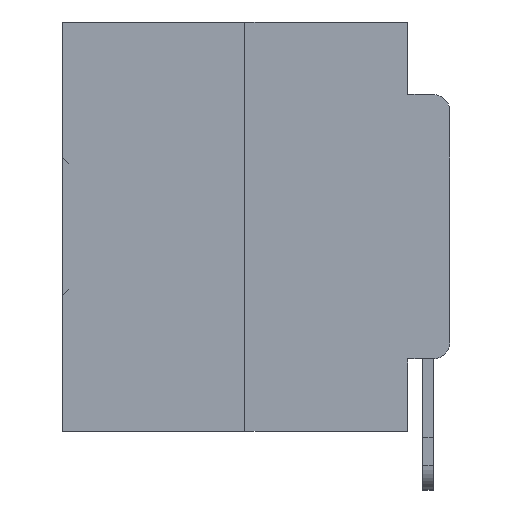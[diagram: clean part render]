
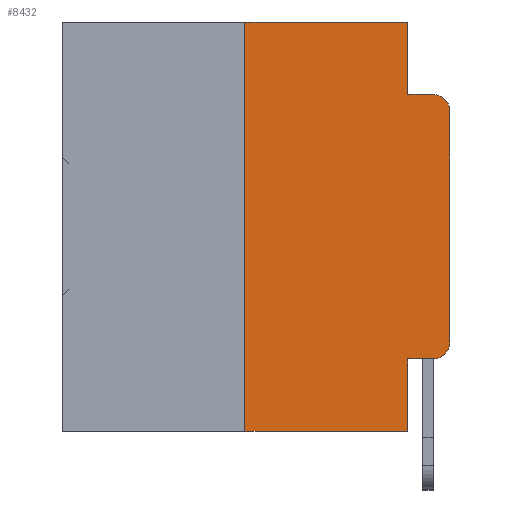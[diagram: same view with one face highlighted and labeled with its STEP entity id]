
A CAD part, left-side view. The second image highlights one B-rep face of the part: STEP entity #8432.
In plain terms, the highlighted planar face has unit normal (-1, 0, 0).
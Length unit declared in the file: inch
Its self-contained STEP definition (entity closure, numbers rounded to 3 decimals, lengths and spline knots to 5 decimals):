
#310 = CARTESIAN_POINT ( 'NONE',  ( 0., 0.473, 0. ) ) ;
#440 = DIRECTION ( 'NONE',  ( 0., 0., -1. ) ) ;
#893 = CARTESIAN_POINT ( 'NONE',  ( 0., 0., 0. ) ) ;
#908 = VERTEX_POINT ( 'NONE', #3097 ) ;
#1462 = CARTESIAN_POINT ( 'NONE',  ( 0., 0.02, -0.1085 ) ) ;
#2169 = ORIENTED_EDGE ( 'NONE', *, *, #18929, .F. ) ;
#3097 = CARTESIAN_POINT ( 'NONE',  ( 0., 0., -0.3915 ) ) ;
#3182 = DIRECTION ( 'NONE',  ( 1., 0., 0. ) ) ;
#3212 = DIRECTION ( 'NONE',  ( 0., -1., 0. ) ) ;
#3274 = ORIENTED_EDGE ( 'NONE', *, *, #28466, .T. ) ;
#3740 = DIRECTION ( 'NONE',  ( 0., 0., 1. ) ) ;
#4311 = DIRECTION ( 'NONE',  ( 0., 0., -1. ) ) ;
#4549 = CARTESIAN_POINT ( 'NONE',  ( 0., 0.051, 0. ) ) ;
#4976 = ORIENTED_EDGE ( 'NONE', *, *, #17083, .F. ) ;
#5153 = VERTEX_POINT ( 'NONE', #35256 ) ;
#5606 = DIRECTION ( 'NONE',  ( 0., -1., 0. ) ) ;
#5955 = CARTESIAN_POINT ( 'NONE',  ( 0., 0.25, 0. ) ) ;
#6010 = LINE ( 'NONE', #14475, #27039 ) ;
#7073 = CARTESIAN_POINT ( 'NONE',  ( 0., 0.051, -0.0885 ) ) ;
#7370 = DIRECTION ( 'NONE',  ( -1., 0., 0. ) ) ;
#7690 = ORIENTED_EDGE ( 'NONE', *, *, #12234, .F. ) ;
#8172 = VERTEX_POINT ( 'NONE', #31947 ) ;
#8432 = ADVANCED_FACE ( 'NONE', ( #31484 ), #33073, .F. ) ;
#9915 = DIRECTION ( 'NONE',  ( 0., -1., 0. ) ) ;
#10198 = ORIENTED_EDGE ( 'NONE', *, *, #22091, .T. ) ;
#10309 = EDGE_CURVE ( 'NONE', #22016, #10993, #26444, .T. ) ;
#10993 = VERTEX_POINT ( 'NONE', #33402 ) ;
#11069 = VECTOR ( 'NONE', #3212, 39.37008 ) ;
#11459 = DIRECTION ( 'NONE',  ( 0., 0., -1. ) ) ;
#11576 = DIRECTION ( 'NONE',  ( 0., 0., 1. ) ) ;
#11639 = ORIENTED_EDGE ( 'NONE', *, *, #15289, .T. ) ;
#12204 = ORIENTED_EDGE ( 'NONE', *, *, #10309, .T. ) ;
#12234 = EDGE_CURVE ( 'NONE', #34002, #23517, #28386, .T. ) ;
#12989 = CIRCLE ( 'NONE', #17070, 0.02 ) ;
#12990 = ORIENTED_EDGE ( 'NONE', *, *, #20644, .F. ) ;
#13266 = CARTESIAN_POINT ( 'NONE',  ( 0., 0.473, -0.5 ) ) ;
#13388 = CARTESIAN_POINT ( 'NONE',  ( 0., 0.051, -0.0885 ) ) ;
#13579 = VERTEX_POINT ( 'NONE', #4549 ) ;
#13599 = LINE ( 'NONE', #27549, #34909 ) ;
#14023 = VECTOR ( 'NONE', #9915, 39.37008 ) ;
#14372 = VECTOR ( 'NONE', #3740, 39.37008 ) ;
#14475 = CARTESIAN_POINT ( 'NONE',  ( 0., 0.051, 0. ) ) ;
#15289 = EDGE_CURVE ( 'NONE', #908, #8172, #28723, .T. ) ;
#16059 = DIRECTION ( 'NONE',  ( 0., -1., 0. ) ) ;
#16426 = EDGE_CURVE ( 'NONE', #13579, #34002, #6010, .T. ) ;
#17070 = AXIS2_PLACEMENT_3D ( 'NONE', #23861, #7370, #11459 ) ;
#17083 = EDGE_CURVE ( 'NONE', #22016, #24878, #22803, .T. ) ;
#17811 = EDGE_CURVE ( 'NONE', #8172, #23517, #33086, .T. ) ;
#18929 = EDGE_CURVE ( 'NONE', #23051, #5153, #27285, .T. ) ;
#19375 = AXIS2_PLACEMENT_3D ( 'NONE', #1462, #20924, #4311 ) ;
#19951 = DIRECTION ( 'NONE',  ( 0., 0., -1. ) ) ;
#20644 = EDGE_CURVE ( 'NONE', #5153, #13579, #13599, .T. ) ;
#20827 = CARTESIAN_POINT ( 'NONE',  ( 0., 0.051, -0.4115 ) ) ;
#20924 = DIRECTION ( 'NONE',  ( -1., 0., 0. ) ) ;
#20940 = AXIS2_PLACEMENT_3D ( 'NONE', #310, #3182, #22556 ) ;
#22016 = VERTEX_POINT ( 'NONE', #20827 ) ;
#22091 = EDGE_CURVE ( 'NONE', #10993, #908, #12989, .T. ) ;
#22556 = DIRECTION ( 'NONE',  ( 0., 0., -1. ) ) ;
#22589 = CARTESIAN_POINT ( 'NONE',  ( 0., 0.051, -0.4115 ) ) ;
#22803 = LINE ( 'NONE', #33273, #34337 ) ;
#22873 = LINE ( 'NONE', #13266, #28300 ) ;
#23051 = VERTEX_POINT ( 'NONE', #33756 ) ;
#23517 = VERTEX_POINT ( 'NONE', #23985 ) ;
#23861 = CARTESIAN_POINT ( 'NONE',  ( 0., 0.02, -0.3915 ) ) ;
#23985 = CARTESIAN_POINT ( 'NONE',  ( 0., 0.02, -0.0885 ) ) ;
#24256 = CARTESIAN_POINT ( 'NONE',  ( 0., 0.051, -0.5 ) ) ;
#24878 = VERTEX_POINT ( 'NONE', #24256 ) ;
#26155 = ORIENTED_EDGE ( 'NONE', *, *, #17811, .T. ) ;
#26444 = LINE ( 'NONE', #22589, #11069 ) ;
#27039 = VECTOR ( 'NONE', #440, 39.37008 ) ;
#27285 = LINE ( 'NONE', #5955, #28108 ) ;
#27549 = CARTESIAN_POINT ( 'NONE',  ( 0., 0.473, 0. ) ) ;
#28108 = VECTOR ( 'NONE', #11576, 39.37008 ) ;
#28300 = VECTOR ( 'NONE', #16059, 39.37008 ) ;
#28386 = LINE ( 'NONE', #7073, #14023 ) ;
#28466 = EDGE_CURVE ( 'NONE', #23051, #24878, #22873, .T. ) ;
#28723 = LINE ( 'NONE', #893, #14372 ) ;
#29769 = EDGE_LOOP ( 'NONE', ( #11639, #26155, #7690, #31097, #12990, #2169, #3274, #4976, #12204, #10198 ) ) ;
#31097 = ORIENTED_EDGE ( 'NONE', *, *, #16426, .F. ) ;
#31484 = FACE_OUTER_BOUND ( 'NONE', #29769, .T. ) ;
#31947 = CARTESIAN_POINT ( 'NONE',  ( 0., 0., -0.1085 ) ) ;
#33073 = PLANE ( 'NONE',  #20940 ) ;
#33086 = CIRCLE ( 'NONE', #19375, 0.02 ) ;
#33273 = CARTESIAN_POINT ( 'NONE',  ( 0., 0.051, 0. ) ) ;
#33402 = CARTESIAN_POINT ( 'NONE',  ( 0., 0.02, -0.4115 ) ) ;
#33756 = CARTESIAN_POINT ( 'NONE',  ( 0., 0.25, -0.5 ) ) ;
#34002 = VERTEX_POINT ( 'NONE', #13388 ) ;
#34337 = VECTOR ( 'NONE', #19951, 39.37008 ) ;
#34909 = VECTOR ( 'NONE', #5606, 39.37008 ) ;
#35256 = CARTESIAN_POINT ( 'NONE',  ( 0., 0.25, 0. ) ) ;
